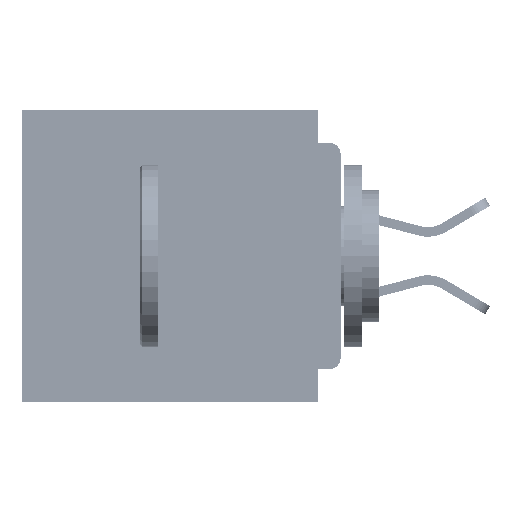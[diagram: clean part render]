
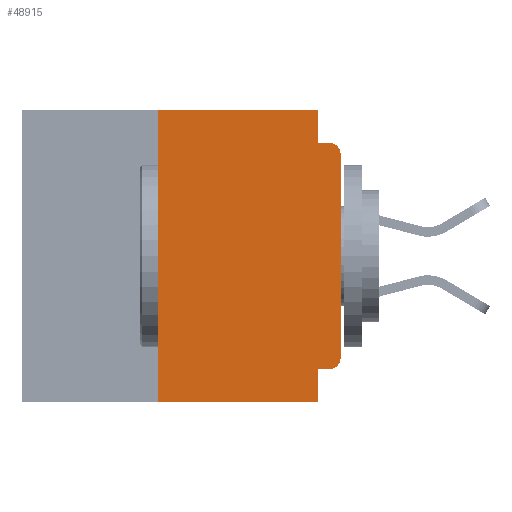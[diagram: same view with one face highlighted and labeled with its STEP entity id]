
A CAD part, left-side view. The second image highlights one B-rep face of the part: STEP entity #48915.
In plain terms, the highlighted planar face has unit normal (-1, 0, 0).
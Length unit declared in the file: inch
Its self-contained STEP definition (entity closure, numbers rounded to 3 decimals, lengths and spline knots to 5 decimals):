
#706 = LINE ( 'NONE', #54673, #60353 ) ;
#783 = EDGE_CURVE ( 'NONE', #46962, #11910, #36468, .T. ) ;
#2095 = ORIENTED_EDGE ( 'NONE', *, *, #28044, .F. ) ;
#3502 = ORIENTED_EDGE ( 'NONE', *, *, #23916, .F. ) ;
#3605 = ORIENTED_EDGE ( 'NONE', *, *, #783, .T. ) ;
#3631 = EDGE_CURVE ( 'NONE', #17019, #9670, #40591, .T. ) ;
#4541 = CARTESIAN_POINT ( 'NONE',  ( 0., 0., -0.355 ) ) ;
#4743 = CARTESIAN_POINT ( 'NONE',  ( 0., 0.015, -0.06 ) ) ;
#7158 = ORIENTED_EDGE ( 'NONE', *, *, #3631, .F. ) ;
#7256 = LINE ( 'NONE', #10077, #8758 ) ;
#8658 = EDGE_LOOP ( 'NONE', ( #51081, #48462, #2095, #17155, #3502, #7158, #23687, #49318, #57450, #3605 ) ) ;
#8758 = VECTOR ( 'NONE', #33762, 39.37008 ) ;
#9498 = DIRECTION ( 'NONE',  ( 0., 0., -1. ) ) ;
#9670 = VERTEX_POINT ( 'NONE', #11952 ) ;
#10077 = CARTESIAN_POINT ( 'NONE',  ( 0., 0.437, 0. ) ) ;
#10393 = DIRECTION ( 'NONE',  ( 0., 0., 1. ) ) ;
#10853 = CARTESIAN_POINT ( 'NONE',  ( 0., 0.25, -0.4 ) ) ;
#11084 = AXIS2_PLACEMENT_3D ( 'NONE', #49960, #45459, #17332 ) ;
#11910 = VERTEX_POINT ( 'NONE', #32781 ) ;
#11952 = CARTESIAN_POINT ( 'NONE',  ( 0., 0.25, 0. ) ) ;
#11958 = CARTESIAN_POINT ( 'NONE',  ( 0., 0.031, 0. ) ) ;
#12563 = PLANE ( 'NONE',  #11084 ) ;
#13875 = VERTEX_POINT ( 'NONE', #52466 ) ;
#15338 = VERTEX_POINT ( 'NONE', #36116 ) ;
#15389 = DIRECTION ( 'NONE',  ( 0., -1., 0. ) ) ;
#17019 = VERTEX_POINT ( 'NONE', #58558 ) ;
#17155 = ORIENTED_EDGE ( 'NONE', *, *, #34699, .F. ) ;
#17332 = DIRECTION ( 'NONE',  ( 0., 0., -1. ) ) ;
#18481 = CARTESIAN_POINT ( 'NONE',  ( 0., 0.031, -0.355 ) ) ;
#19868 = LINE ( 'NONE', #54975, #54344 ) ;
#20929 = LINE ( 'NONE', #22889, #44391 ) ;
#21373 = VECTOR ( 'NONE', #59080, 39.37008 ) ;
#21862 = VERTEX_POINT ( 'NONE', #50984 ) ;
#22889 = CARTESIAN_POINT ( 'NONE',  ( 0., 0., 0. ) ) ;
#23687 = ORIENTED_EDGE ( 'NONE', *, *, #34619, .T. ) ;
#23916 = EDGE_CURVE ( 'NONE', #9670, #37984, #7256, .T. ) ;
#27261 = VERTEX_POINT ( 'NONE', #42188 ) ;
#27593 = DIRECTION ( 'NONE',  ( 0., 0., 1. ) ) ;
#28044 = EDGE_CURVE ( 'NONE', #15338, #27261, #38394, .T. ) ;
#28160 = VECTOR ( 'NONE', #10393, 39.37008 ) ;
#28477 = VERTEX_POINT ( 'NONE', #18481 ) ;
#29403 = CARTESIAN_POINT ( 'NONE',  ( 0., 0., -0.045 ) ) ;
#31011 = CARTESIAN_POINT ( 'NONE',  ( 0., 0.437, -0.4 ) ) ;
#31331 = DIRECTION ( 'NONE',  ( 0., 0., -1. ) ) ;
#32781 = CARTESIAN_POINT ( 'NONE',  ( 0., 0., -0.34 ) ) ;
#32825 = DIRECTION ( 'NONE',  ( 0., 1., 0. ) ) ;
#32899 = AXIS2_PLACEMENT_3D ( 'NONE', #45178, #45045, #44520 ) ;
#33762 = DIRECTION ( 'NONE',  ( 0., -1., 0. ) ) ;
#33829 = LINE ( 'NONE', #31011, #21373 ) ;
#34619 = EDGE_CURVE ( 'NONE', #17019, #21862, #33829, .T. ) ;
#34699 = EDGE_CURVE ( 'NONE', #37984, #15338, #19868, .T. ) ;
#36116 = CARTESIAN_POINT ( 'NONE',  ( 0., 0.031, -0.045 ) ) ;
#36323 = DIRECTION ( 'NONE',  ( 0., 0., -1. ) ) ;
#36468 = CIRCLE ( 'NONE', #32899, 0.015 ) ;
#37654 = EDGE_CURVE ( 'NONE', #13875, #27261, #50559, .T. ) ;
#37680 = DIRECTION ( 'NONE',  ( -1., 0., 0. ) ) ;
#37984 = VERTEX_POINT ( 'NONE', #11958 ) ;
#38394 = LINE ( 'NONE', #29403, #50880 ) ;
#39906 = EDGE_CURVE ( 'NONE', #11910, #13875, #20929, .T. ) ;
#40591 = LINE ( 'NONE', #10853, #28160 ) ;
#42188 = CARTESIAN_POINT ( 'NONE',  ( 0., 0.015, -0.045 ) ) ;
#44033 = EDGE_CURVE ( 'NONE', #46962, #28477, #47723, .T. ) ;
#44391 = VECTOR ( 'NONE', #27593, 39.37008 ) ;
#44520 = DIRECTION ( 'NONE',  ( 0., 0., -1. ) ) ;
#45045 = DIRECTION ( 'NONE',  ( -1., 0., 0. ) ) ;
#45178 = CARTESIAN_POINT ( 'NONE',  ( 0., 0.015, -0.34 ) ) ;
#45459 = DIRECTION ( 'NONE',  ( 1., 0., 0. ) ) ;
#46962 = VERTEX_POINT ( 'NONE', #52830 ) ;
#47723 = LINE ( 'NONE', #4541, #49212 ) ;
#47898 = FACE_OUTER_BOUND ( 'NONE', #8658, .T. ) ;
#48462 = ORIENTED_EDGE ( 'NONE', *, *, #37654, .T. ) ;
#48910 = EDGE_CURVE ( 'NONE', #28477, #21862, #706, .T. ) ;
#48915 = ADVANCED_FACE ( 'NONE', ( #47898 ), #12563, .F. ) ;
#49212 = VECTOR ( 'NONE', #32825, 39.37008 ) ;
#49318 = ORIENTED_EDGE ( 'NONE', *, *, #48910, .F. ) ;
#49960 = CARTESIAN_POINT ( 'NONE',  ( 0., 0.437, 0. ) ) ;
#50559 = CIRCLE ( 'NONE', #51050, 0.015 ) ;
#50880 = VECTOR ( 'NONE', #15389, 39.37008 ) ;
#50984 = CARTESIAN_POINT ( 'NONE',  ( 0., 0.031, -0.4 ) ) ;
#51050 = AXIS2_PLACEMENT_3D ( 'NONE', #4743, #37680, #9498 ) ;
#51081 = ORIENTED_EDGE ( 'NONE', *, *, #39906, .T. ) ;
#52466 = CARTESIAN_POINT ( 'NONE',  ( 0., 0., -0.06 ) ) ;
#52830 = CARTESIAN_POINT ( 'NONE',  ( 0., 0.015, -0.355 ) ) ;
#54344 = VECTOR ( 'NONE', #36323, 39.37008 ) ;
#54673 = CARTESIAN_POINT ( 'NONE',  ( 0., 0.031, -0.4 ) ) ;
#54975 = CARTESIAN_POINT ( 'NONE',  ( 0., 0.031, 0. ) ) ;
#57450 = ORIENTED_EDGE ( 'NONE', *, *, #44033, .F. ) ;
#58558 = CARTESIAN_POINT ( 'NONE',  ( 0., 0.25, -0.4 ) ) ;
#59080 = DIRECTION ( 'NONE',  ( 0., -1., 0. ) ) ;
#60353 = VECTOR ( 'NONE', #31331, 39.37008 ) ;
